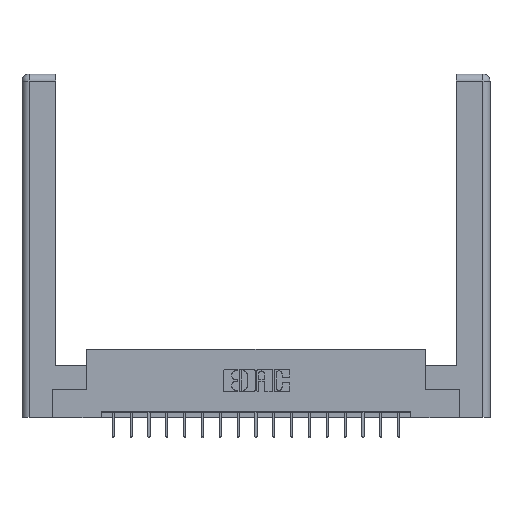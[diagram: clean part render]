
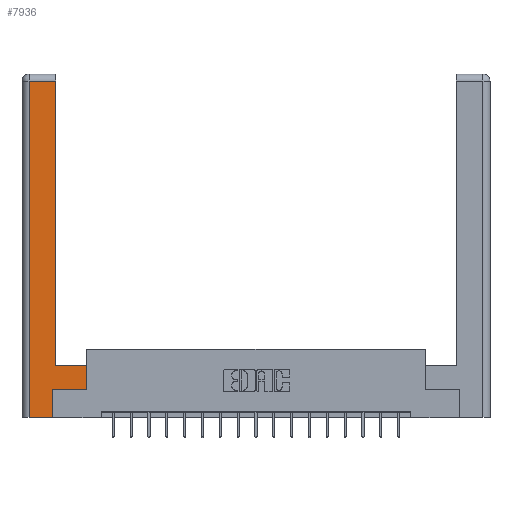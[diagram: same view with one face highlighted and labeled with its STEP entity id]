
A CAD part, top view. The second image highlights one B-rep face of the part: STEP entity #7936.
In plain terms, the highlighted planar face has unit normal (0, 0, 1).
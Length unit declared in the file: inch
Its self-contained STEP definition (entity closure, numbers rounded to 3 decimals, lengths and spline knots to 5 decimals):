
#178 = LINE ( 'NONE', #18166, #15415 ) ;
#179 = EDGE_CURVE ( 'NONE', #6890, #5041, #7473, .T. ) ;
#188 = VERTEX_POINT ( 'NONE', #10315 ) ;
#200 = VECTOR ( 'NONE', #17764, 39.37008 ) ;
#352 = CARTESIAN_POINT ( 'NONE',  ( 0., 0., 0. ) ) ;
#1288 = ORIENTED_EDGE ( 'NONE', *, *, #12199, .T. ) ;
#1366 = EDGE_CURVE ( 'NONE', #5041, #6682, #11942, .T. ) ;
#1801 = DIRECTION ( 'NONE',  ( 1., 0., 0. ) ) ;
#1969 = VECTOR ( 'NONE', #8174, 39.37008 ) ;
#1996 = EDGE_CURVE ( 'NONE', #14084, #7708, #11428, .T. ) ;
#3175 = DIRECTION ( 'NONE',  ( 0., 1., 0. ) ) ;
#3929 = ORIENTED_EDGE ( 'NONE', *, *, #179, .T. ) ;
#3988 = CARTESIAN_POINT ( 'NONE',  ( 0.565, 0.45, 0. ) ) ;
#4003 = CARTESIAN_POINT ( 'NONE',  ( 0.265, 0., 0. ) ) ;
#4191 = CARTESIAN_POINT ( 'NONE',  ( 0.0615, 0., 0. ) ) ;
#4466 = DIRECTION ( 'NONE',  ( 0., 1., 0. ) ) ;
#5041 = VERTEX_POINT ( 'NONE', #8299 ) ;
#5150 = VECTOR ( 'NONE', #13204, 39.37008 ) ;
#5994 = DIRECTION ( 'NONE',  ( -1., 0., 0. ) ) ;
#6092 = LINE ( 'NONE', #7131, #5150 ) ;
#6326 = VECTOR ( 'NONE', #11599, 39.37008 ) ;
#6682 = VERTEX_POINT ( 'NONE', #15921 ) ;
#6890 = VERTEX_POINT ( 'NONE', #12595 ) ;
#7131 = CARTESIAN_POINT ( 'NONE',  ( 0.0615, 0., 0. ) ) ;
#7148 = FACE_OUTER_BOUND ( 'NONE', #8300, .T. ) ;
#7329 = VECTOR ( 'NONE', #3175, 39.37008 ) ;
#7473 = LINE ( 'NONE', #3988, #6326 ) ;
#7579 = LINE ( 'NONE', #12012, #7329 ) ;
#7708 = VERTEX_POINT ( 'NONE', #14173 ) ;
#7869 = VECTOR ( 'NONE', #12350, 39.37008 ) ;
#7936 = ADVANCED_FACE ( 'NONE', ( #7148 ), #10567, .F. ) ;
#8174 = DIRECTION ( 'NONE',  ( -1., 0., 0. ) ) ;
#8266 = ORIENTED_EDGE ( 'NONE', *, *, #1366, .T. ) ;
#8299 = CARTESIAN_POINT ( 'NONE',  ( 0.565, 0.45, 0. ) ) ;
#8300 = EDGE_LOOP ( 'NONE', ( #13893, #16789, #1288, #9651, #16456, #13979, #3929, #8266 ) ) ;
#8532 = CARTESIAN_POINT ( 'NONE',  ( 0.295, 2.94, 0. ) ) ;
#9566 = AXIS2_PLACEMENT_3D ( 'NONE', #352, #14817, #5994 ) ;
#9651 = ORIENTED_EDGE ( 'NONE', *, *, #11067, .T. ) ;
#10315 = CARTESIAN_POINT ( 'NONE',  ( 0.265, 0.245, 0. ) ) ;
#10521 = VERTEX_POINT ( 'NONE', #4191 ) ;
#10567 = PLANE ( 'NONE',  #9566 ) ;
#10874 = LINE ( 'NONE', #18288, #7869 ) ;
#11025 = CARTESIAN_POINT ( 'NONE',  ( 0.0615, 2.94, 0. ) ) ;
#11067 = EDGE_CURVE ( 'NONE', #10521, #13825, #178, .T. ) ;
#11428 = LINE ( 'NONE', #11025, #1969 ) ;
#11452 = EDGE_CURVE ( 'NONE', #13825, #188, #14027, .T. ) ;
#11599 = DIRECTION ( 'NONE',  ( 0., 1., 0. ) ) ;
#11917 = CARTESIAN_POINT ( 'NONE',  ( 0.295, 0.45, 0. ) ) ;
#11942 = LINE ( 'NONE', #11917, #200 ) ;
#12012 = CARTESIAN_POINT ( 'NONE',  ( 0.295, 3., 0. ) ) ;
#12199 = EDGE_CURVE ( 'NONE', #7708, #10521, #6092, .T. ) ;
#12350 = DIRECTION ( 'NONE',  ( 1., 0., 0. ) ) ;
#12595 = CARTESIAN_POINT ( 'NONE',  ( 0.565, 0.245, 0. ) ) ;
#13204 = DIRECTION ( 'NONE',  ( 0., -1., 0. ) ) ;
#13250 = CARTESIAN_POINT ( 'NONE',  ( 0.265, 0.245, 0. ) ) ;
#13269 = EDGE_CURVE ( 'NONE', #188, #6890, #10874, .T. ) ;
#13472 = EDGE_CURVE ( 'NONE', #6682, #14084, #7579, .T. ) ;
#13825 = VERTEX_POINT ( 'NONE', #4003 ) ;
#13893 = ORIENTED_EDGE ( 'NONE', *, *, #13472, .T. ) ;
#13979 = ORIENTED_EDGE ( 'NONE', *, *, #13269, .T. ) ;
#14027 = LINE ( 'NONE', #13250, #15632 ) ;
#14084 = VERTEX_POINT ( 'NONE', #8532 ) ;
#14173 = CARTESIAN_POINT ( 'NONE',  ( 0.0615, 2.94, 0. ) ) ;
#14817 = DIRECTION ( 'NONE',  ( 0., 0., -1. ) ) ;
#15415 = VECTOR ( 'NONE', #1801, 39.37008 ) ;
#15632 = VECTOR ( 'NONE', #4466, 39.37008 ) ;
#15921 = CARTESIAN_POINT ( 'NONE',  ( 0.295, 0.45, 0. ) ) ;
#16456 = ORIENTED_EDGE ( 'NONE', *, *, #11452, .T. ) ;
#16789 = ORIENTED_EDGE ( 'NONE', *, *, #1996, .T. ) ;
#17764 = DIRECTION ( 'NONE',  ( -1., 0., 0. ) ) ;
#18166 = CARTESIAN_POINT ( 'NONE',  ( 0.265, 0., 0. ) ) ;
#18288 = CARTESIAN_POINT ( 'NONE',  ( 0.565, 0.245, 0. ) ) ;
